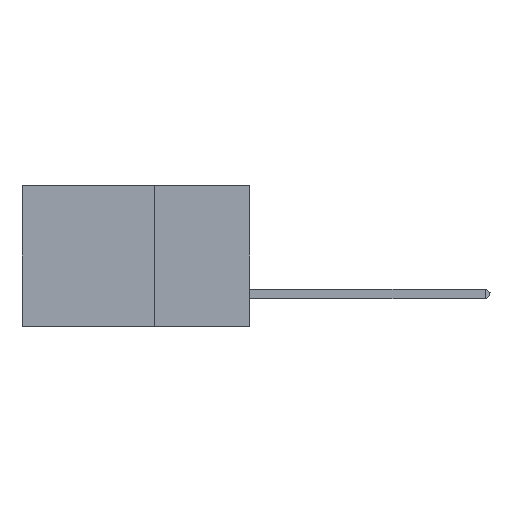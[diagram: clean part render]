
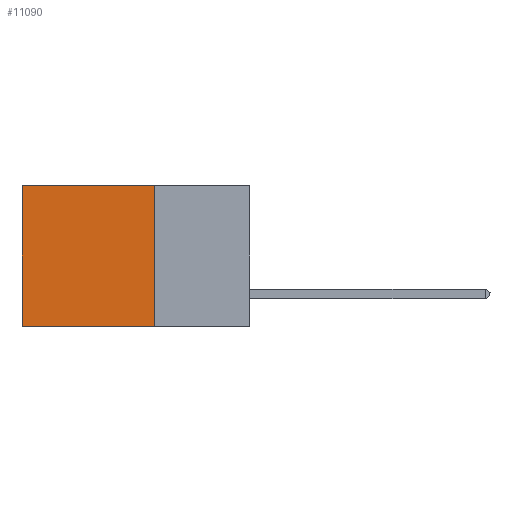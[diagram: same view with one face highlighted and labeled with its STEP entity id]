
A CAD part, left-side view. The second image highlights one B-rep face of the part: STEP entity #11090.
In plain terms, the highlighted planar face has unit normal (-1, 0, 0).
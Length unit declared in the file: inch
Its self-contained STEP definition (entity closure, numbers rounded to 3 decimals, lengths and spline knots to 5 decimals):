
#1801 = CARTESIAN_POINT ( 'NONE',  ( 0.2875, 0.25, 0. ) ) ;
#1815 = DIRECTION ( 'NONE',  ( 0., 0., -1. ) ) ;
#2672 = VERTEX_POINT ( 'NONE', #33042 ) ;
#5103 = DIRECTION ( 'NONE',  ( 1., 0., 0. ) ) ;
#6026 = LINE ( 'NONE', #1801, #25941 ) ;
#6598 = ORIENTED_EDGE ( 'NONE', *, *, #44012, .F. ) ;
#9497 = CARTESIAN_POINT ( 'NONE',  ( 0.2875, 0.6, 0. ) ) ;
#10033 = EDGE_CURVE ( 'NONE', #13098, #45599, #42398, .T. ) ;
#10034 = LINE ( 'NONE', #24665, #38251 ) ;
#11090 = ADVANCED_FACE ( 'NONE', ( #11633 ), #44121, .F. ) ;
#11633 = FACE_OUTER_BOUND ( 'NONE', #23469, .T. ) ;
#12891 = CARTESIAN_POINT ( 'NONE',  ( 0.2875, 0.25, 0. ) ) ;
#13098 = VERTEX_POINT ( 'NONE', #9497 ) ;
#15553 = CARTESIAN_POINT ( 'NONE',  ( 0.2875, 0.25, 0. ) ) ;
#15629 = VECTOR ( 'NONE', #42780, 39.37008 ) ;
#16654 = ORIENTED_EDGE ( 'NONE', *, *, #43756, .F. ) ;
#17438 = CARTESIAN_POINT ( 'NONE',  ( 0.2875, 0.25, 0. ) ) ;
#22635 = DIRECTION ( 'NONE',  ( 0., 0., -1. ) ) ;
#23469 = EDGE_LOOP ( 'NONE', ( #39322, #6598, #16654, #31688 ) ) ;
#24127 = EDGE_CURVE ( 'NONE', #26860, #13098, #6026, .T. ) ;
#24665 = CARTESIAN_POINT ( 'NONE',  ( 0.2875, 0.25, -0.37 ) ) ;
#25941 = VECTOR ( 'NONE', #44634, 39.37008 ) ;
#26860 = VERTEX_POINT ( 'NONE', #12891 ) ;
#31688 = ORIENTED_EDGE ( 'NONE', *, *, #24127, .T. ) ;
#32234 = DIRECTION ( 'NONE',  ( 0., 1., 0. ) ) ;
#33042 = CARTESIAN_POINT ( 'NONE',  ( 0.2875, 0.25, -0.37 ) ) ;
#34275 = CARTESIAN_POINT ( 'NONE',  ( 0.2875, 0.6, 0. ) ) ;
#38251 = VECTOR ( 'NONE', #32234, 39.37008 ) ;
#39322 = ORIENTED_EDGE ( 'NONE', *, *, #10033, .T. ) ;
#39476 = LINE ( 'NONE', #15553, #15629 ) ;
#41142 = VECTOR ( 'NONE', #22635, 39.37008 ) ;
#42398 = LINE ( 'NONE', #34275, #41142 ) ;
#42780 = DIRECTION ( 'NONE',  ( 0., 0., -1. ) ) ;
#43756 = EDGE_CURVE ( 'NONE', #26860, #2672, #39476, .T. ) ;
#44012 = EDGE_CURVE ( 'NONE', #2672, #45599, #10034, .T. ) ;
#44121 = PLANE ( 'NONE',  #49368 ) ;
#44634 = DIRECTION ( 'NONE',  ( 0., 1., 0. ) ) ;
#44981 = CARTESIAN_POINT ( 'NONE',  ( 0.2875, 0.6, -0.37 ) ) ;
#45599 = VERTEX_POINT ( 'NONE', #44981 ) ;
#49368 = AXIS2_PLACEMENT_3D ( 'NONE', #17438, #5103, #1815 ) ;
